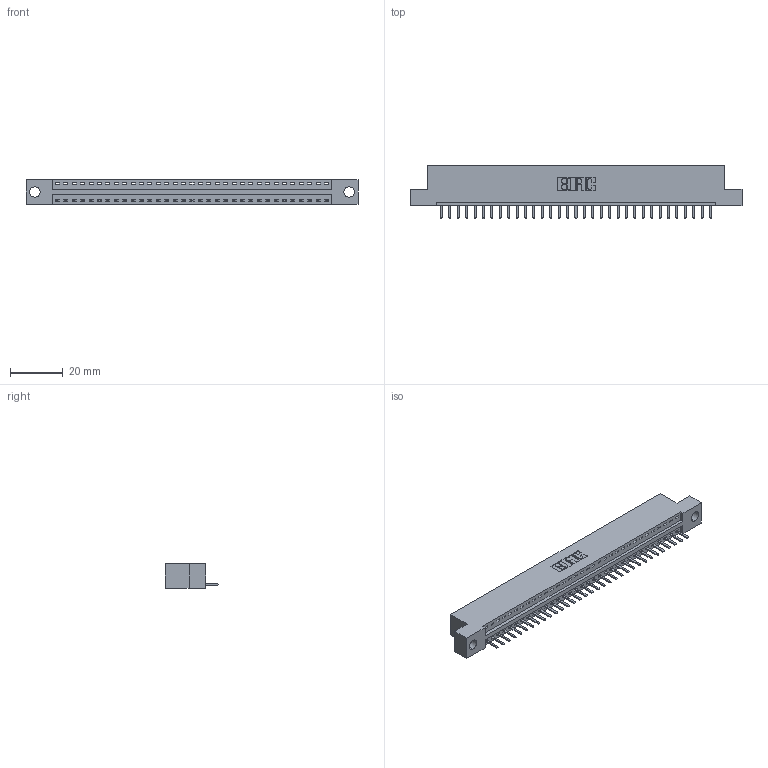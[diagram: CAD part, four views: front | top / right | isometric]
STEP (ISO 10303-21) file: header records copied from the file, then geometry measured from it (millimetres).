
FILE_DESCRIPTION (( 'STEP AP203' ), '1' );
FILE_NAME ('396-033-520-104.STEP', '2018-09-05T12:31:07', ( '' ), ( '' ), 'SwSTEP 2.0', 'SolidWorks 2016', '' );
FILE_SCHEMA (( 'CONFIG_CONTROL_DESIGN' ));
Length unit declared in the file: inch
Products named in the file (3): 345-292-001_345-293-120; 396-033-520-104; 346 Part_Flush Mounting Lugs - 0.156 Dia-TH
Assembly tree (34 placements, depth 2):
  396-033-520-104
    346 Part_Flush Mounting Lugs - 0.156 Dia-TH
    345-292-001_345-293-120  x33
Bounding box: 125.35 x 20.02 x 9.4 mm (x, y, z)
Volume: 11753.9 mm3; surface area: 14081.8 mm2
Topology: 34 solids, 34 shells, 2168 faces, 6401 edges, 4178 vertices
Faces by surface type: plane 1462, cylinder 706
Entity records: 21809 total; most frequent: CARTESIAN_POINT 3759, ORIENTED_EDGE 3714, DIRECTION 3315, EDGE_CURVE 1857, VECTOR 1589, LINE 1589, VERTEX_POINT 1234, AXIS2_PLACEMENT_3D 863
